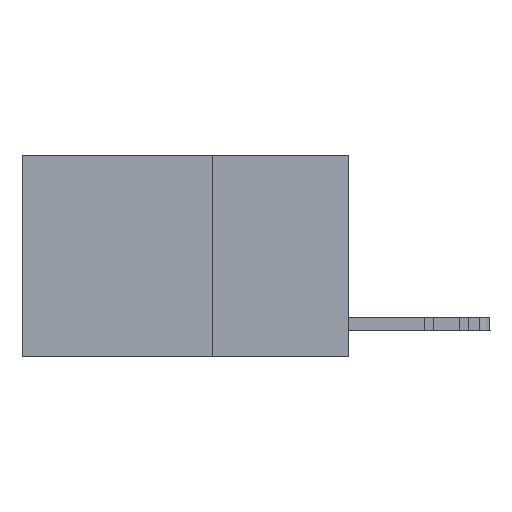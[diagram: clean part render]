
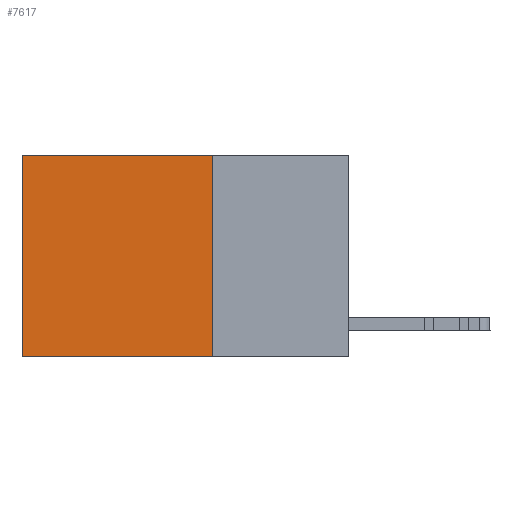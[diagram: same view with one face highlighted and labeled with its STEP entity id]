
A CAD part, left-side view. The second image highlights one B-rep face of the part: STEP entity #7617.
In plain terms, the highlighted planar face has unit normal (-1, 0, 0).
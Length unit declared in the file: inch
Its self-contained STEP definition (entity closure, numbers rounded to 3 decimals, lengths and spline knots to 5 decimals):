
#754 = LINE ( 'NONE', #3060, #9448 ) ;
#2271 = CARTESIAN_POINT ( 'NONE',  ( 0.2625, 0.6, 0. ) ) ;
#3060 = CARTESIAN_POINT ( 'NONE',  ( 0.2625, 0.25, 0. ) ) ;
#3688 = DIRECTION ( 'NONE',  ( 0., 1., 0. ) ) ;
#3803 = DIRECTION ( 'NONE',  ( 0., 1., 0. ) ) ;
#4824 = VERTEX_POINT ( 'NONE', #26420 ) ;
#6009 = EDGE_LOOP ( 'NONE', ( #28116, #18290, #19529, #14113 ) ) ;
#7016 = VERTEX_POINT ( 'NONE', #2271 ) ;
#7617 = ADVANCED_FACE ( 'NONE', ( #28623 ), #8749, .F. ) ;
#7867 = LINE ( 'NONE', #12647, #21152 ) ;
#8749 = PLANE ( 'NONE',  #19866 ) ;
#9448 = VECTOR ( 'NONE', #9739, 39.37008 ) ;
#9739 = DIRECTION ( 'NONE',  ( 0., 0., -1. ) ) ;
#10599 = CARTESIAN_POINT ( 'NONE',  ( 0.2625, 0.6, 0. ) ) ;
#11004 = EDGE_CURVE ( 'NONE', #14453, #4824, #754, .T. ) ;
#11183 = CARTESIAN_POINT ( 'NONE',  ( 0.2625, 0.25, 0. ) ) ;
#11652 = DIRECTION ( 'NONE',  ( 1., 0., 0. ) ) ;
#12647 = CARTESIAN_POINT ( 'NONE',  ( 0.2625, 0.25, 0. ) ) ;
#14113 = ORIENTED_EDGE ( 'NONE', *, *, #27297, .T. ) ;
#14229 = CARTESIAN_POINT ( 'NONE',  ( 0.2625, 0.25, 0. ) ) ;
#14337 = EDGE_CURVE ( 'NONE', #7016, #17316, #17266, .T. ) ;
#14453 = VERTEX_POINT ( 'NONE', #11183 ) ;
#15233 = DIRECTION ( 'NONE',  ( 0., 0., -1. ) ) ;
#15613 = VECTOR ( 'NONE', #15233, 39.37008 ) ;
#17266 = LINE ( 'NONE', #10599, #15613 ) ;
#17316 = VERTEX_POINT ( 'NONE', #21637 ) ;
#18290 = ORIENTED_EDGE ( 'NONE', *, *, #22165, .F. ) ;
#18868 = DIRECTION ( 'NONE',  ( 0., 0., -1. ) ) ;
#19529 = ORIENTED_EDGE ( 'NONE', *, *, #11004, .F. ) ;
#19866 = AXIS2_PLACEMENT_3D ( 'NONE', #14229, #11652, #18868 ) ;
#20555 = VECTOR ( 'NONE', #3803, 39.37008 ) ;
#21152 = VECTOR ( 'NONE', #3688, 39.37008 ) ;
#21331 = CARTESIAN_POINT ( 'NONE',  ( 0.2625, 0.25, -0.37 ) ) ;
#21637 = CARTESIAN_POINT ( 'NONE',  ( 0.2625, 0.6, -0.37 ) ) ;
#22165 = EDGE_CURVE ( 'NONE', #4824, #17316, #23502, .T. ) ;
#23502 = LINE ( 'NONE', #21331, #20555 ) ;
#26420 = CARTESIAN_POINT ( 'NONE',  ( 0.2625, 0.25, -0.37 ) ) ;
#27297 = EDGE_CURVE ( 'NONE', #14453, #7016, #7867, .T. ) ;
#28116 = ORIENTED_EDGE ( 'NONE', *, *, #14337, .T. ) ;
#28623 = FACE_OUTER_BOUND ( 'NONE', #6009, .T. ) ;
